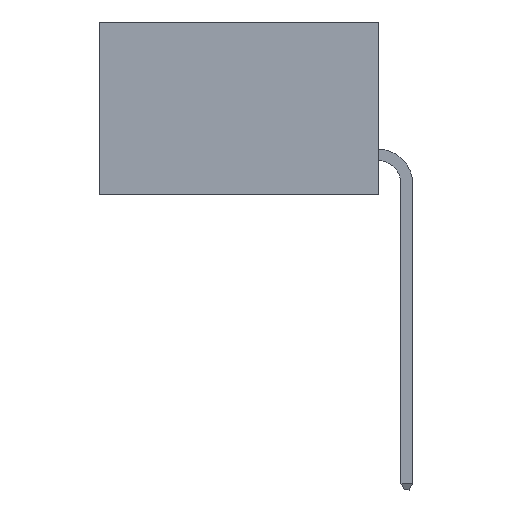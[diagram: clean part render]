
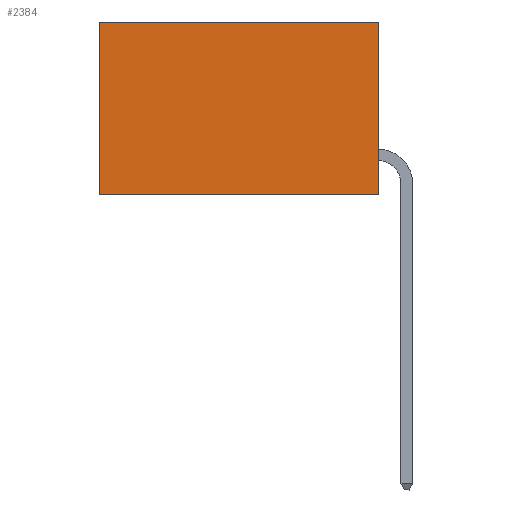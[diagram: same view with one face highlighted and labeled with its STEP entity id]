
A CAD part, left-side view. The second image highlights one B-rep face of the part: STEP entity #2384.
In plain terms, the highlighted planar face has unit normal (-1, 0, 0).
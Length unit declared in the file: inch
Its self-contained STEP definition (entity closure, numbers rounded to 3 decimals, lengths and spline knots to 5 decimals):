
#15 = VERTEX_POINT ( 'NONE', #6989 ) ;
#47 = LINE ( 'NONE', #7703, #1783 ) ;
#615 = LINE ( 'NONE', #3823, #4201 ) ;
#672 = EDGE_CURVE ( 'NONE', #966, #8806, #1705, .T. ) ;
#891 = PLANE ( 'NONE',  #6711 ) ;
#895 = ORIENTED_EDGE ( 'NONE', *, *, #2932, .F. ) ;
#966 = VERTEX_POINT ( 'NONE', #6215 ) ;
#1209 = FACE_OUTER_BOUND ( 'NONE', #5745, .T. ) ;
#1705 = LINE ( 'NONE', #7490, #8726 ) ;
#1774 = EDGE_CURVE ( 'NONE', #15, #8806, #615, .T. ) ;
#1783 = VECTOR ( 'NONE', #8672, 39.37008 ) ;
#2384 = ADVANCED_FACE ( 'NONE', ( #1209 ), #891, .F. ) ;
#2932 = EDGE_CURVE ( 'NONE', #3951, #966, #47, .T. ) ;
#3090 = ORIENTED_EDGE ( 'NONE', *, *, #6644, .T. ) ;
#3242 = DIRECTION ( 'NONE',  ( 0., 1., 0. ) ) ;
#3569 = DIRECTION ( 'NONE',  ( 0., 0., -1. ) ) ;
#3823 = CARTESIAN_POINT ( 'NONE',  ( 0.298, 0.6, 0. ) ) ;
#3951 = VERTEX_POINT ( 'NONE', #7984 ) ;
#4201 = VECTOR ( 'NONE', #3569, 39.37008 ) ;
#4386 = LINE ( 'NONE', #5765, #7743 ) ;
#5444 = DIRECTION ( 'NONE',  ( 0., 1., 0. ) ) ;
#5745 = EDGE_LOOP ( 'NONE', ( #8440, #6506, #895, #3090 ) ) ;
#5765 = CARTESIAN_POINT ( 'NONE',  ( 0.298, 0., 0. ) ) ;
#6215 = CARTESIAN_POINT ( 'NONE',  ( 0.298, 0., -0.37 ) ) ;
#6506 = ORIENTED_EDGE ( 'NONE', *, *, #672, .F. ) ;
#6644 = EDGE_CURVE ( 'NONE', #3951, #15, #4386, .T. ) ;
#6711 = AXIS2_PLACEMENT_3D ( 'NONE', #7059, #7879, #8775 ) ;
#6847 = CARTESIAN_POINT ( 'NONE',  ( 0.298, 0.6, -0.37 ) ) ;
#6989 = CARTESIAN_POINT ( 'NONE',  ( 0.298, 0.6, 0. ) ) ;
#7059 = CARTESIAN_POINT ( 'NONE',  ( 0.298, 0., 0. ) ) ;
#7490 = CARTESIAN_POINT ( 'NONE',  ( 0.298, 0., -0.37 ) ) ;
#7703 = CARTESIAN_POINT ( 'NONE',  ( 0.298, 0., 0. ) ) ;
#7743 = VECTOR ( 'NONE', #5444, 39.37008 ) ;
#7879 = DIRECTION ( 'NONE',  ( 1., 0., 0. ) ) ;
#7984 = CARTESIAN_POINT ( 'NONE',  ( 0.298, 0., 0. ) ) ;
#8440 = ORIENTED_EDGE ( 'NONE', *, *, #1774, .T. ) ;
#8672 = DIRECTION ( 'NONE',  ( 0., 0., -1. ) ) ;
#8726 = VECTOR ( 'NONE', #3242, 39.37008 ) ;
#8775 = DIRECTION ( 'NONE',  ( 0., 0., -1. ) ) ;
#8806 = VERTEX_POINT ( 'NONE', #6847 ) ;
